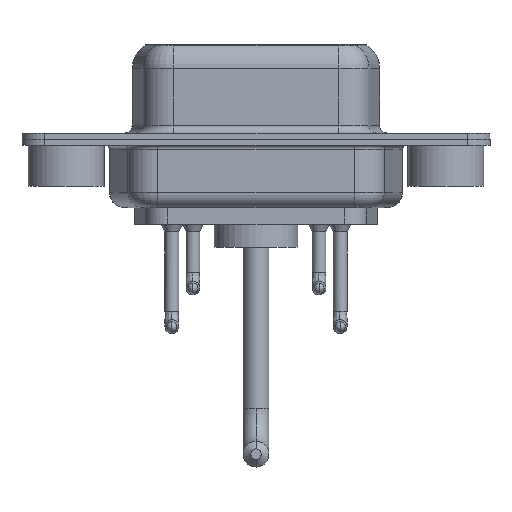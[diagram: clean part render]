
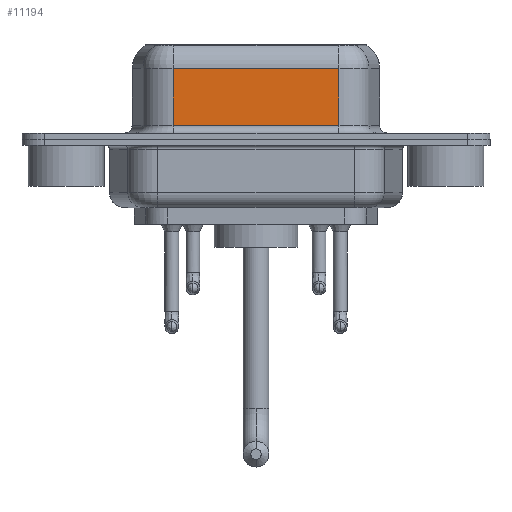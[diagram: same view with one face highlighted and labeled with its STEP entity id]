
A CAD part, front view. The second image highlights one B-rep face of the part: STEP entity #11194.
In plain terms, the highlighted planar face has unit normal (0, -1, 0).
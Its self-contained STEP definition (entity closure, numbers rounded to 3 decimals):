
#264 = VECTOR ( 'NONE', #13621, 1000. ) ;
#458 = DIRECTION ( 'NONE',  ( -1., 0., 0. ) ) ;
#2035 = CARTESIAN_POINT ( 'NONE',  ( 17.962, -3.95, 6.4 ) ) ;
#2327 = VERTEX_POINT ( 'NONE', #3949 ) ;
#2345 = CARTESIAN_POINT ( 'NONE',  ( 17.962, -3.95, 4.65 ) ) ;
#3215 = DIRECTION ( 'NONE',  ( 0., 0., -1. ) ) ;
#3372 = LINE ( 'NONE', #9642, #8121 ) ;
#3412 = AXIS2_PLACEMENT_3D ( 'NONE', #7933, #12983, #458 ) ;
#3701 = ORIENTED_EDGE ( 'NONE', *, *, #11495, .T. ) ;
#3754 = CARTESIAN_POINT ( 'NONE',  ( 17.962, -3.95, 0.9 ) ) ;
#3949 = CARTESIAN_POINT ( 'NONE',  ( 17.962, -3.95, 4.65 ) ) ;
#4461 = EDGE_CURVE ( 'NONE', #5877, #7192, #4984, .T. ) ;
#4806 = VERTEX_POINT ( 'NONE', #9355 ) ;
#4984 = LINE ( 'NONE', #3754, #11290 ) ;
#5069 = DIRECTION ( 'NONE',  ( 1., 0., 0. ) ) ;
#5372 = EDGE_CURVE ( 'NONE', #4806, #5877, #3372, .T. ) ;
#5877 = VERTEX_POINT ( 'NONE', #10942 ) ;
#6535 = FACE_OUTER_BOUND ( 'NONE', #11722, .T. ) ;
#6692 = CARTESIAN_POINT ( 'NONE',  ( 17.962, -3.95, 0.9 ) ) ;
#7192 = VERTEX_POINT ( 'NONE', #6692 ) ;
#7933 = CARTESIAN_POINT ( 'NONE',  ( 17.962, -3.95, 6.4 ) ) ;
#8121 = VECTOR ( 'NONE', #3215, 1000. ) ;
#8651 = ORIENTED_EDGE ( 'NONE', *, *, #10825, .F. ) ;
#9355 = CARTESIAN_POINT ( 'NONE',  ( 7.038, -3.95, 4.65 ) ) ;
#9642 = CARTESIAN_POINT ( 'NONE',  ( 7.038, -3.95, 6.4 ) ) ;
#9718 = ORIENTED_EDGE ( 'NONE', *, *, #5372, .T. ) ;
#9847 = LINE ( 'NONE', #2345, #264 ) ;
#10825 = EDGE_CURVE ( 'NONE', #2327, #7192, #13312, .T. ) ;
#10942 = CARTESIAN_POINT ( 'NONE',  ( 7.038, -3.95, 0.9 ) ) ;
#11194 = ADVANCED_FACE ( 'NONE', ( #6535 ), #11592, .F. ) ;
#11280 = ORIENTED_EDGE ( 'NONE', *, *, #4461, .T. ) ;
#11290 = VECTOR ( 'NONE', #5069, 1000. ) ;
#11495 = EDGE_CURVE ( 'NONE', #2327, #4806, #9847, .T. ) ;
#11592 = PLANE ( 'NONE',  #3412 ) ;
#11722 = EDGE_LOOP ( 'NONE', ( #8651, #3701, #9718, #11280 ) ) ;
#12983 = DIRECTION ( 'NONE',  ( 0., 1., 0. ) ) ;
#13312 = LINE ( 'NONE', #2035, #14745 ) ;
#13621 = DIRECTION ( 'NONE',  ( -1., 0., 0. ) ) ;
#14527 = DIRECTION ( 'NONE',  ( 0., 0., -1. ) ) ;
#14745 = VECTOR ( 'NONE', #14527, 1000. ) ;
